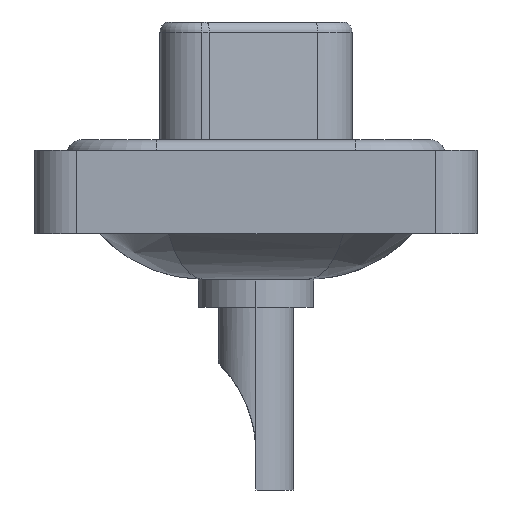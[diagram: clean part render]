
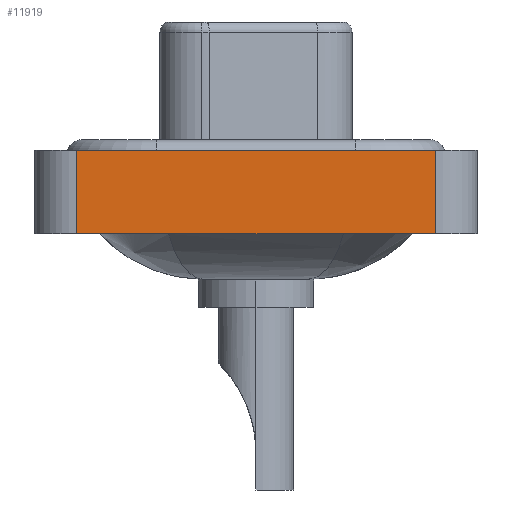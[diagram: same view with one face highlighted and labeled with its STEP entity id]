
A CAD part, left-side view. The second image highlights one B-rep face of the part: STEP entity #11919.
In plain terms, the highlighted planar face has unit normal (-1, 0, 0).
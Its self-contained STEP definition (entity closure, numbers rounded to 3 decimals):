
#560 = AXIS2_PLACEMENT_3D ( 'NONE', #8838, #4728, #13978 ) ;
#628 = ORIENTED_EDGE ( 'NONE', *, *, #14111, .F. ) ;
#869 = VERTEX_POINT ( 'NONE', #8051 ) ;
#1650 = EDGE_CURVE ( 'NONE', #869, #5208, #9549, .T. ) ;
#1869 = ORIENTED_EDGE ( 'NONE', *, *, #5436, .F. ) ;
#3383 = LINE ( 'NONE', #15177, #6247 ) ;
#4082 = EDGE_CURVE ( 'NONE', #5208, #14021, #3383, .T. ) ;
#4728 = DIRECTION ( 'NONE',  ( -1., 0., 0. ) ) ;
#4754 = CARTESIAN_POINT ( 'NONE',  ( -7.3, -8.55, 0.4 ) ) ;
#4890 = ORIENTED_EDGE ( 'NONE', *, *, #1650, .T. ) ;
#5208 = VERTEX_POINT ( 'NONE', #8548 ) ;
#5436 = EDGE_CURVE ( 'NONE', #6049, #14021, #12824, .T. ) ;
#6049 = VERTEX_POINT ( 'NONE', #7423 ) ;
#6247 = VECTOR ( 'NONE', #12310, 1000. ) ;
#7423 = CARTESIAN_POINT ( 'NONE',  ( -7.3, 8.55, 0.4 ) ) ;
#7472 = VECTOR ( 'NONE', #15782, 1000. ) ;
#8051 = CARTESIAN_POINT ( 'NONE',  ( -7.3, 8.55, -3.6 ) ) ;
#8283 = CARTESIAN_POINT ( 'NONE',  ( -7.3, -8.55, -3.6 ) ) ;
#8302 = CARTESIAN_POINT ( 'NONE',  ( -7.3, -8.55, 0.4 ) ) ;
#8548 = CARTESIAN_POINT ( 'NONE',  ( -7.3, -8.55, -3.6 ) ) ;
#8783 = DIRECTION ( 'NONE',  ( 0., -1., 0. ) ) ;
#8838 = CARTESIAN_POINT ( 'NONE',  ( -7.3, -8.55, -3.6 ) ) ;
#9549 = LINE ( 'NONE', #8283, #7472 ) ;
#10140 = EDGE_LOOP ( 'NONE', ( #15567, #1869, #628, #4890 ) ) ;
#10586 = VECTOR ( 'NONE', #8783, 1000. ) ;
#11819 = VECTOR ( 'NONE', #12040, 1000. ) ;
#11919 = ADVANCED_FACE ( 'NONE', ( #16520 ), #15240, .T. ) ;
#12040 = DIRECTION ( 'NONE',  ( 0., 0., 1. ) ) ;
#12310 = DIRECTION ( 'NONE',  ( 0., 0., 1. ) ) ;
#12824 = LINE ( 'NONE', #4754, #10586 ) ;
#13309 = LINE ( 'NONE', #15753, #11819 ) ;
#13978 = DIRECTION ( 'NONE',  ( 0., 0., 1. ) ) ;
#14021 = VERTEX_POINT ( 'NONE', #8302 ) ;
#14111 = EDGE_CURVE ( 'NONE', #869, #6049, #13309, .T. ) ;
#15177 = CARTESIAN_POINT ( 'NONE',  ( -7.3, -8.55, -3.6 ) ) ;
#15240 = PLANE ( 'NONE',  #560 ) ;
#15567 = ORIENTED_EDGE ( 'NONE', *, *, #4082, .T. ) ;
#15753 = CARTESIAN_POINT ( 'NONE',  ( -7.3, 8.55, -3.6 ) ) ;
#15782 = DIRECTION ( 'NONE',  ( 0., -1., 0. ) ) ;
#16520 = FACE_OUTER_BOUND ( 'NONE', #10140, .T. ) ;
